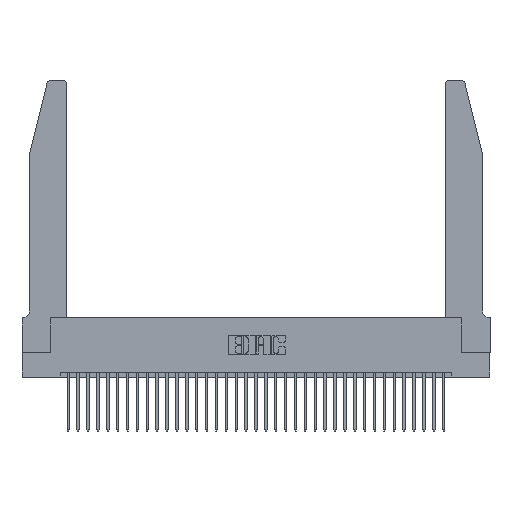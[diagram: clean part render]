
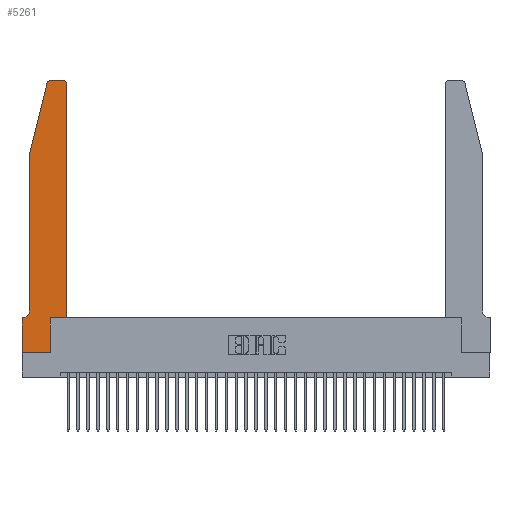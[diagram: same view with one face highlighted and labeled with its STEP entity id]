
A CAD part, top view. The second image highlights one B-rep face of the part: STEP entity #5261.
In plain terms, the highlighted planar face has unit normal (0, 0, 1).
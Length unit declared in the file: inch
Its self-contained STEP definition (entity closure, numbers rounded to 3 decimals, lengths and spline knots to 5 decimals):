
#69 = VECTOR ( 'NONE', #10021, 39.37008 ) ;
#380 = CIRCLE ( 'NONE', #11414, 0.03 ) ;
#1187 = LINE ( 'NONE', #34420, #34503 ) ;
#1262 = CARTESIAN_POINT ( 'NONE',  ( 0.0055, 0.42, 0.37 ) ) ;
#1893 = VERTEX_POINT ( 'NONE', #8634 ) ;
#2189 = VECTOR ( 'NONE', #27454, 39.37008 ) ;
#2389 = ORIENTED_EDGE ( 'NONE', *, *, #22553, .T. ) ;
#2571 = VERTEX_POINT ( 'NONE', #16862 ) ;
#4430 = VECTOR ( 'NONE', #5744, 39.37008 ) ;
#5154 = EDGE_CURVE ( 'NONE', #6653, #9953, #35671, .T. ) ;
#5261 = ADVANCED_FACE ( 'NONE', ( #33931 ), #10543, .T. ) ;
#5263 = EDGE_LOOP ( 'NONE', ( #33671, #32603, #21130, #31073, #8751, #10817, #2389, #35253, #7839, #11342, #26709, #30395 ) ) ;
#5744 = DIRECTION ( 'NONE',  ( 1., 0., 0. ) ) ;
#5960 = VERTEX_POINT ( 'NONE', #15771 ) ;
#6545 = DIRECTION ( 'NONE',  ( -1., 0., 0. ) ) ;
#6574 = DIRECTION ( 'NONE',  ( 0., 0., -1. ) ) ;
#6653 = VERTEX_POINT ( 'NONE', #27461 ) ;
#6966 = DIRECTION ( 'NONE',  ( -0.239, -0.971, 0. ) ) ;
#7550 = EDGE_CURVE ( 'NONE', #26079, #23909, #15150, .T. ) ;
#7692 = AXIS2_PLACEMENT_3D ( 'NONE', #1262, #6574, #9370 ) ;
#7839 = ORIENTED_EDGE ( 'NONE', *, *, #7898, .T. ) ;
#7898 = EDGE_CURVE ( 'NONE', #9953, #14567, #34610, .T. ) ;
#8337 = CARTESIAN_POINT ( 'NONE',  ( 0.4505, 0.35, 0.37 ) ) ;
#8386 = VERTEX_POINT ( 'NONE', #12642 ) ;
#8634 = CARTESIAN_POINT ( 'NONE',  ( 0.4505, 2.72, 0.37 ) ) ;
#8677 = EDGE_CURVE ( 'NONE', #23178, #8386, #12498, .T. ) ;
#8751 = ORIENTED_EDGE ( 'NONE', *, *, #31596, .T. ) ;
#8900 = CARTESIAN_POINT ( 'NONE',  ( 0.284, 2.72, 0.37 ) ) ;
#9370 = DIRECTION ( 'NONE',  ( -1., 0., 0. ) ) ;
#9556 = EDGE_CURVE ( 'NONE', #23909, #23178, #18460, .T. ) ;
#9953 = VERTEX_POINT ( 'NONE', #23443 ) ;
#10021 = DIRECTION ( 'NONE',  ( 0., 1., 0. ) ) ;
#10543 = PLANE ( 'NONE',  #25303 ) ;
#10768 = DIRECTION ( 'NONE',  ( 0., 0., 1. ) ) ;
#10817 = ORIENTED_EDGE ( 'NONE', *, *, #18488, .T. ) ;
#10892 = CARTESIAN_POINT ( 'NONE',  ( 0., 0.35, 0.37 ) ) ;
#11149 = LINE ( 'NONE', #8337, #14144 ) ;
#11154 = CARTESIAN_POINT ( 'NONE',  ( 0., 0., 0.37 ) ) ;
#11342 = ORIENTED_EDGE ( 'NONE', *, *, #29175, .T. ) ;
#11414 = AXIS2_PLACEMENT_3D ( 'NONE', #19003, #30593, #25165 ) ;
#11590 = VECTOR ( 'NONE', #29608, 39.37008 ) ;
#11723 = VERTEX_POINT ( 'NONE', #24178 ) ;
#12498 = LINE ( 'NONE', #28806, #14244 ) ;
#12642 = CARTESIAN_POINT ( 'NONE',  ( 0.0755, 0.42, 0.37 ) ) ;
#12965 = VECTOR ( 'NONE', #6545, 39.37008 ) ;
#13049 = CARTESIAN_POINT ( 'NONE',  ( 0.2865, 0.35, 0.37 ) ) ;
#13421 = DIRECTION ( 'NONE',  ( 1., 0., 0. ) ) ;
#13489 = EDGE_CURVE ( 'NONE', #5960, #26079, #1187, .T. ) ;
#14144 = VECTOR ( 'NONE', #19745, 39.37008 ) ;
#14244 = VECTOR ( 'NONE', #23034, 39.37008 ) ;
#14266 = LINE ( 'NONE', #24690, #2189 ) ;
#14554 = VECTOR ( 'NONE', #6966, 39.37008 ) ;
#14567 = VERTEX_POINT ( 'NONE', #20231 ) ;
#14921 = CARTESIAN_POINT ( 'NONE',  ( 0.0755, 2., 0.37 ) ) ;
#15150 = CIRCLE ( 'NONE', #34851, 0.03 ) ;
#15771 = CARTESIAN_POINT ( 'NONE',  ( 0.4205, 2.75, 0.37 ) ) ;
#16242 = VERTEX_POINT ( 'NONE', #16408 ) ;
#16408 = CARTESIAN_POINT ( 'NONE',  ( 0.0055, 0.35, 0.37 ) ) ;
#16815 = LINE ( 'NONE', #31178, #12965 ) ;
#16862 = CARTESIAN_POINT ( 'NONE',  ( 0., 0.35, 0.37 ) ) ;
#17175 = DIRECTION ( 'NONE',  ( 0., 0., 1. ) ) ;
#18460 = LINE ( 'NONE', #14921, #14554 ) ;
#18488 = EDGE_CURVE ( 'NONE', #16242, #2571, #16815, .T. ) ;
#19003 = CARTESIAN_POINT ( 'NONE',  ( 0.4205, 2.72, 0.37 ) ) ;
#19745 = DIRECTION ( 'NONE',  ( 1., 0., 0. ) ) ;
#20231 = CARTESIAN_POINT ( 'NONE',  ( 0.2865, 0.35, 0.37 ) ) ;
#21130 = ORIENTED_EDGE ( 'NONE', *, *, #9556, .T. ) ;
#22047 = EDGE_CURVE ( 'NONE', #1893, #5960, #380, .T. ) ;
#22321 = CARTESIAN_POINT ( 'NONE',  ( 0.0755, 2., 0.37 ) ) ;
#22553 = EDGE_CURVE ( 'NONE', #2571, #6653, #31943, .T. ) ;
#23034 = DIRECTION ( 'NONE',  ( 0., -1., 0. ) ) ;
#23178 = VERTEX_POINT ( 'NONE', #22321 ) ;
#23443 = CARTESIAN_POINT ( 'NONE',  ( 0.2865, 0., 0.37 ) ) ;
#23909 = VERTEX_POINT ( 'NONE', #32956 ) ;
#24175 = CARTESIAN_POINT ( 'NONE',  ( 0., 0., 0.37 ) ) ;
#24178 = CARTESIAN_POINT ( 'NONE',  ( 0.4505, 0.35, 0.37 ) ) ;
#24690 = CARTESIAN_POINT ( 'NONE',  ( 0.4505, 0.35, 0.37 ) ) ;
#25165 = DIRECTION ( 'NONE',  ( 1., 0., 0. ) ) ;
#25303 = AXIS2_PLACEMENT_3D ( 'NONE', #10892, #10768, #13421 ) ;
#26079 = VERTEX_POINT ( 'NONE', #29533 ) ;
#26177 = DIRECTION ( 'NONE',  ( -1., 0., 0. ) ) ;
#26709 = ORIENTED_EDGE ( 'NONE', *, *, #27445, .T. ) ;
#27445 = EDGE_CURVE ( 'NONE', #11723, #1893, #14266, .T. ) ;
#27454 = DIRECTION ( 'NONE',  ( 0., 1., 0. ) ) ;
#27461 = CARTESIAN_POINT ( 'NONE',  ( 0., 0., 0.37 ) ) ;
#28313 = DIRECTION ( 'NONE',  ( 1., 0., 0. ) ) ;
#28806 = CARTESIAN_POINT ( 'NONE',  ( 0.0755, 2., 0.37 ) ) ;
#29175 = EDGE_CURVE ( 'NONE', #14567, #11723, #11149, .T. ) ;
#29533 = CARTESIAN_POINT ( 'NONE',  ( 0.284, 2.75, 0.37 ) ) ;
#29608 = DIRECTION ( 'NONE',  ( 0., -1., 0. ) ) ;
#30395 = ORIENTED_EDGE ( 'NONE', *, *, #22047, .T. ) ;
#30593 = DIRECTION ( 'NONE',  ( 0., 0., 1. ) ) ;
#31073 = ORIENTED_EDGE ( 'NONE', *, *, #8677, .T. ) ;
#31178 = CARTESIAN_POINT ( 'NONE',  ( 0.0755, 0.35, 0.37 ) ) ;
#31596 = EDGE_CURVE ( 'NONE', #8386, #16242, #35752, .T. ) ;
#31943 = LINE ( 'NONE', #24175, #11590 ) ;
#32603 = ORIENTED_EDGE ( 'NONE', *, *, #7550, .T. ) ;
#32956 = CARTESIAN_POINT ( 'NONE',  ( 0.25487, 2.72718, 0.37 ) ) ;
#33671 = ORIENTED_EDGE ( 'NONE', *, *, #13489, .T. ) ;
#33931 = FACE_OUTER_BOUND ( 'NONE', #5263, .T. ) ;
#34420 = CARTESIAN_POINT ( 'NONE',  ( 0.2605, 2.75, 0.37 ) ) ;
#34503 = VECTOR ( 'NONE', #26177, 39.37008 ) ;
#34610 = LINE ( 'NONE', #13049, #69 ) ;
#34851 = AXIS2_PLACEMENT_3D ( 'NONE', #8900, #17175, #28313 ) ;
#35253 = ORIENTED_EDGE ( 'NONE', *, *, #5154, .T. ) ;
#35671 = LINE ( 'NONE', #11154, #4430 ) ;
#35752 = CIRCLE ( 'NONE', #7692, 0.07 ) ;
